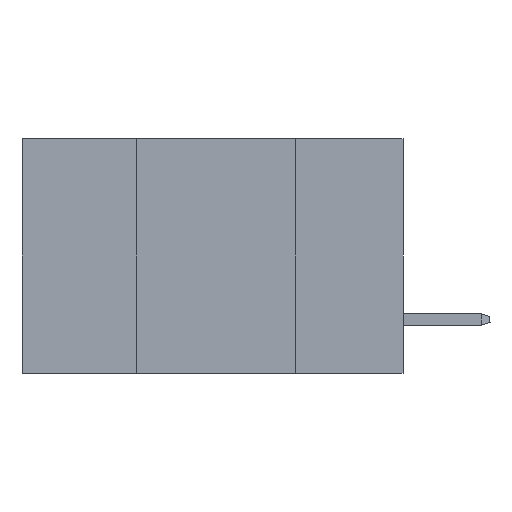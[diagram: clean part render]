
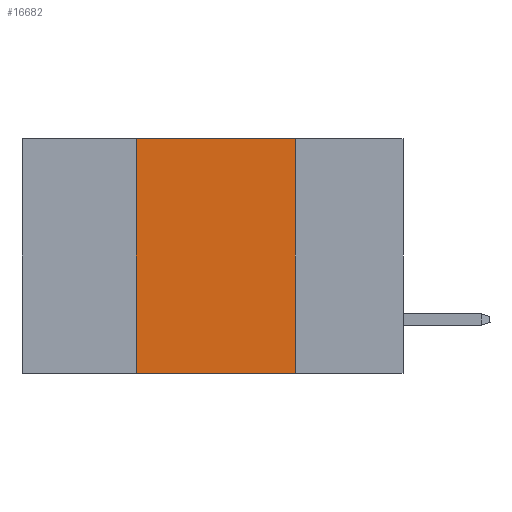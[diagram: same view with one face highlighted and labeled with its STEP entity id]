
A CAD part, left-side view. The second image highlights one B-rep face of the part: STEP entity #16682.
In plain terms, the highlighted planar face has unit normal (-1, 0, 0).
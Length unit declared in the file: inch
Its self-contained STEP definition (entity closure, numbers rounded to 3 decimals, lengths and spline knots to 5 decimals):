
#1326 = PLANE ( 'NONE',  #24200 ) ;
#1460 = VECTOR ( 'NONE', #6251, 39.37008 ) ;
#3538 = LINE ( 'NONE', #8641, #1460 ) ;
#4076 = CARTESIAN_POINT ( 'NONE',  ( 0., 0.17, 0. ) ) ;
#4178 = CARTESIAN_POINT ( 'NONE',  ( 0., 0.42, 0. ) ) ;
#6251 = DIRECTION ( 'NONE',  ( 0., 0., -1. ) ) ;
#6304 = ORIENTED_EDGE ( 'NONE', *, *, #16961, .F. ) ;
#6690 = CARTESIAN_POINT ( 'NONE',  ( 0., 0.6, 0. ) ) ;
#6896 = ORIENTED_EDGE ( 'NONE', *, *, #11511, .F. ) ;
#6935 = DIRECTION ( 'NONE',  ( 1., 0., 0. ) ) ;
#8641 = CARTESIAN_POINT ( 'NONE',  ( 0., 0.17, 0. ) ) ;
#11511 = EDGE_CURVE ( 'NONE', #26568, #33675, #3538, .T. ) ;
#12246 = LINE ( 'NONE', #15120, #25019 ) ;
#12728 = LINE ( 'NONE', #17036, #19051 ) ;
#14137 = VERTEX_POINT ( 'NONE', #4178 ) ;
#14809 = CARTESIAN_POINT ( 'NONE',  ( 0., 0.42, -0.37 ) ) ;
#14947 = EDGE_CURVE ( 'NONE', #29150, #33675, #12728, .T. ) ;
#15120 = CARTESIAN_POINT ( 'NONE',  ( 0., 0.42, 0. ) ) ;
#16682 = ADVANCED_FACE ( 'NONE', ( #25020 ), #1326, .F. ) ;
#16961 = EDGE_CURVE ( 'NONE', #14137, #26568, #30055, .T. ) ;
#17036 = CARTESIAN_POINT ( 'NONE',  ( 0., 0.6, -0.37 ) ) ;
#19051 = VECTOR ( 'NONE', #23101, 39.37008 ) ;
#19891 = CARTESIAN_POINT ( 'NONE',  ( 0., 0.6, 0. ) ) ;
#23101 = DIRECTION ( 'NONE',  ( 0., -1., 0. ) ) ;
#23595 = DIRECTION ( 'NONE',  ( 0., 0., 1. ) ) ;
#24200 = AXIS2_PLACEMENT_3D ( 'NONE', #19891, #6935, #30458 ) ;
#24223 = VECTOR ( 'NONE', #32103, 39.37008 ) ;
#25019 = VECTOR ( 'NONE', #23595, 39.37008 ) ;
#25020 = FACE_OUTER_BOUND ( 'NONE', #30961, .T. ) ;
#25277 = ORIENTED_EDGE ( 'NONE', *, *, #14947, .T. ) ;
#26568 = VERTEX_POINT ( 'NONE', #4076 ) ;
#26714 = EDGE_CURVE ( 'NONE', #29150, #14137, #12246, .T. ) ;
#28110 = ORIENTED_EDGE ( 'NONE', *, *, #26714, .F. ) ;
#29150 = VERTEX_POINT ( 'NONE', #14809 ) ;
#30055 = LINE ( 'NONE', #6690, #24223 ) ;
#30458 = DIRECTION ( 'NONE',  ( 0., 0., -1. ) ) ;
#30961 = EDGE_LOOP ( 'NONE', ( #6896, #6304, #28110, #25277 ) ) ;
#31078 = CARTESIAN_POINT ( 'NONE',  ( 0., 0.17, -0.37 ) ) ;
#32103 = DIRECTION ( 'NONE',  ( 0., -1., 0. ) ) ;
#33675 = VERTEX_POINT ( 'NONE', #31078 ) ;
